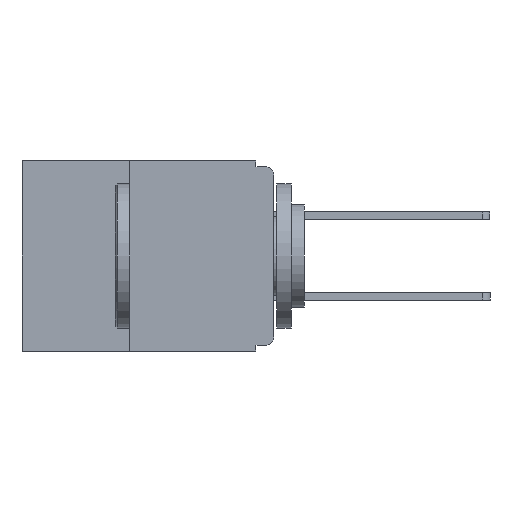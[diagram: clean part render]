
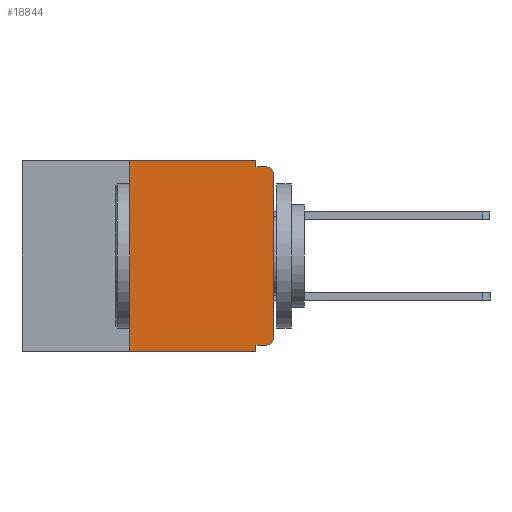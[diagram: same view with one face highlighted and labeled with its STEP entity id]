
A CAD part, left-side view. The second image highlights one B-rep face of the part: STEP entity #18844.
In plain terms, the highlighted planar face has unit normal (-1, 0, 0).
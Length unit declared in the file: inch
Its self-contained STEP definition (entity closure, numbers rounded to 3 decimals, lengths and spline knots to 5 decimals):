
#162 = EDGE_CURVE ( 'NONE', #18142, #1090, #7294, .T. ) ;
#251 = EDGE_CURVE ( 'NONE', #14743, #5602, #5430, .T. ) ;
#496 = AXIS2_PLACEMENT_3D ( 'NONE', #12588, #28696, #14865 ) ;
#716 = VECTOR ( 'NONE', #17768, 39.37008 ) ;
#787 = FACE_OUTER_BOUND ( 'NONE', #21826, .T. ) ;
#1090 = VERTEX_POINT ( 'NONE', #26025 ) ;
#1141 = CARTESIAN_POINT ( 'NONE',  ( 0., 0.437, 0. ) ) ;
#1735 = ORIENTED_EDGE ( 'NONE', *, *, #20188, .T. ) ;
#2264 = ORIENTED_EDGE ( 'NONE', *, *, #15748, .F. ) ;
#2998 = VECTOR ( 'NONE', #14106, 39.37008 ) ;
#3157 = VERTEX_POINT ( 'NONE', #16241 ) ;
#3209 = DIRECTION ( 'NONE',  ( 0., 0., 1. ) ) ;
#3417 = LINE ( 'NONE', #15732, #15230 ) ;
#3497 = LINE ( 'NONE', #1141, #9175 ) ;
#3645 = ORIENTED_EDGE ( 'NONE', *, *, #162, .T. ) ;
#3875 = CARTESIAN_POINT ( 'NONE',  ( 0., 0.031, -0.01 ) ) ;
#4212 = VECTOR ( 'NONE', #3209, 39.37008 ) ;
#4907 = ORIENTED_EDGE ( 'NONE', *, *, #10984, .F. ) ;
#5430 = CIRCLE ( 'NONE', #17498, 0.015 ) ;
#5602 = VERTEX_POINT ( 'NONE', #30296 ) ;
#5666 = DIRECTION ( 'NONE',  ( -1., 0., 0. ) ) ;
#5861 = DIRECTION ( 'NONE',  ( -1., 0., 0. ) ) ;
#6151 = DIRECTION ( 'NONE',  ( 0., -1., 0. ) ) ;
#7294 = LINE ( 'NONE', #8603, #716 ) ;
#8263 = ORIENTED_EDGE ( 'NONE', *, *, #27448, .F. ) ;
#8603 = CARTESIAN_POINT ( 'NONE',  ( 0., 0.437, -0.33 ) ) ;
#8633 = VERTEX_POINT ( 'NONE', #11844 ) ;
#9175 = VECTOR ( 'NONE', #6151, 39.37008 ) ;
#9278 = VECTOR ( 'NONE', #21564, 39.37008 ) ;
#9885 = CARTESIAN_POINT ( 'NONE',  ( 0., 0., -0.01 ) ) ;
#10190 = LINE ( 'NONE', #30110, #2998 ) ;
#10267 = PLANE ( 'NONE',  #496 ) ;
#10402 = ORIENTED_EDGE ( 'NONE', *, *, #27116, .F. ) ;
#10745 = LINE ( 'NONE', #23758, #9278 ) ;
#10984 = EDGE_CURVE ( 'NONE', #13736, #1090, #22209, .T. ) ;
#11844 = CARTESIAN_POINT ( 'NONE',  ( 0., 0., -0.305 ) ) ;
#11856 = EDGE_CURVE ( 'NONE', #8633, #14743, #22149, .T. ) ;
#12002 = LINE ( 'NONE', #9885, #23540 ) ;
#12006 = VERTEX_POINT ( 'NONE', #3875 ) ;
#12588 = CARTESIAN_POINT ( 'NONE',  ( 0., 0.437, 0. ) ) ;
#13736 = VERTEX_POINT ( 'NONE', #21197 ) ;
#14106 = DIRECTION ( 'NONE',  ( 0., 0., 1. ) ) ;
#14139 = CIRCLE ( 'NONE', #18801, 0.015 ) ;
#14743 = VERTEX_POINT ( 'NONE', #15636 ) ;
#14865 = DIRECTION ( 'NONE',  ( 0., 0., -1. ) ) ;
#15230 = VECTOR ( 'NONE', #18080, 39.37008 ) ;
#15636 = CARTESIAN_POINT ( 'NONE',  ( 0., 0., -0.025 ) ) ;
#15732 = CARTESIAN_POINT ( 'NONE',  ( 0., 0.031, 0. ) ) ;
#15748 = EDGE_CURVE ( 'NONE', #20993, #13736, #10745, .T. ) ;
#16241 = CARTESIAN_POINT ( 'NONE',  ( 0., 0.031, 0. ) ) ;
#16443 = CARTESIAN_POINT ( 'NONE',  ( 0., 0.031, -0.33 ) ) ;
#17327 = CARTESIAN_POINT ( 'NONE',  ( 0., 0., 0. ) ) ;
#17498 = AXIS2_PLACEMENT_3D ( 'NONE', #24640, #5666, #22918 ) ;
#17768 = DIRECTION ( 'NONE',  ( 0., -1., 0. ) ) ;
#18080 = DIRECTION ( 'NONE',  ( 0., 0., -1. ) ) ;
#18142 = VERTEX_POINT ( 'NONE', #25751 ) ;
#18801 = AXIS2_PLACEMENT_3D ( 'NONE', #19800, #5861, #22109 ) ;
#18844 = ADVANCED_FACE ( 'NONE', ( #787 ), #10267, .F. ) ;
#19004 = EDGE_CURVE ( 'NONE', #27684, #3157, #3497, .T. ) ;
#19800 = CARTESIAN_POINT ( 'NONE',  ( 0., 0.015, -0.305 ) ) ;
#20188 = EDGE_CURVE ( 'NONE', #20993, #8633, #14139, .T. ) ;
#20993 = VERTEX_POINT ( 'NONE', #26992 ) ;
#21197 = CARTESIAN_POINT ( 'NONE',  ( 0., 0.031, -0.32 ) ) ;
#21494 = VECTOR ( 'NONE', #25785, 39.37008 ) ;
#21564 = DIRECTION ( 'NONE',  ( 0., 1., 0. ) ) ;
#21826 = EDGE_LOOP ( 'NONE', ( #26545, #27089, #8263, #10402, #23922, #25956, #3645, #4907, #2264, #1735 ) ) ;
#22109 = DIRECTION ( 'NONE',  ( 0., 0., -1. ) ) ;
#22149 = LINE ( 'NONE', #17327, #4212 ) ;
#22209 = LINE ( 'NONE', #16443, #21494 ) ;
#22918 = DIRECTION ( 'NONE',  ( 0., 0., -1. ) ) ;
#23540 = VECTOR ( 'NONE', #28330, 39.37008 ) ;
#23758 = CARTESIAN_POINT ( 'NONE',  ( 0., 0., -0.32 ) ) ;
#23922 = ORIENTED_EDGE ( 'NONE', *, *, #19004, .F. ) ;
#24640 = CARTESIAN_POINT ( 'NONE',  ( 0., 0.015, -0.025 ) ) ;
#25751 = CARTESIAN_POINT ( 'NONE',  ( 0., 0.25, -0.33 ) ) ;
#25785 = DIRECTION ( 'NONE',  ( 0., 0., -1. ) ) ;
#25956 = ORIENTED_EDGE ( 'NONE', *, *, #27327, .F. ) ;
#26025 = CARTESIAN_POINT ( 'NONE',  ( 0., 0.031, -0.33 ) ) ;
#26545 = ORIENTED_EDGE ( 'NONE', *, *, #11856, .T. ) ;
#26950 = CARTESIAN_POINT ( 'NONE',  ( 0., 0.25, 0. ) ) ;
#26992 = CARTESIAN_POINT ( 'NONE',  ( 0., 0.015, -0.32 ) ) ;
#27089 = ORIENTED_EDGE ( 'NONE', *, *, #251, .T. ) ;
#27116 = EDGE_CURVE ( 'NONE', #3157, #12006, #3417, .T. ) ;
#27327 = EDGE_CURVE ( 'NONE', #18142, #27684, #10190, .T. ) ;
#27448 = EDGE_CURVE ( 'NONE', #12006, #5602, #12002, .T. ) ;
#27684 = VERTEX_POINT ( 'NONE', #26950 ) ;
#28330 = DIRECTION ( 'NONE',  ( 0., -1., 0. ) ) ;
#28696 = DIRECTION ( 'NONE',  ( 1., 0., 0. ) ) ;
#30110 = CARTESIAN_POINT ( 'NONE',  ( 0., 0.25, -0.33 ) ) ;
#30296 = CARTESIAN_POINT ( 'NONE',  ( 0., 0.015, -0.01 ) ) ;
